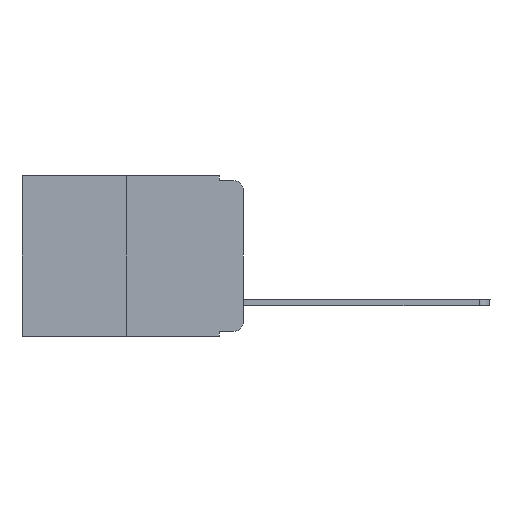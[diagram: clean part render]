
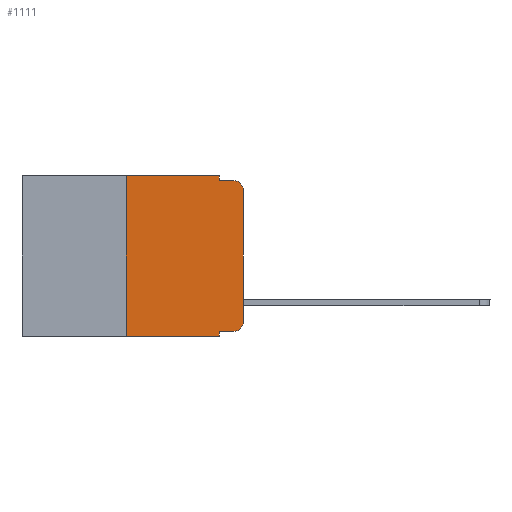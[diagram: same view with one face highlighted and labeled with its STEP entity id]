
A CAD part, left-side view. The second image highlights one B-rep face of the part: STEP entity #1111.
In plain terms, the highlighted planar face has unit normal (-1, 0, 0).
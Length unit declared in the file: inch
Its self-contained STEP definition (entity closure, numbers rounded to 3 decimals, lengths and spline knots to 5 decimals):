
#256 = VERTEX_POINT ( 'NONE', #7959 ) ;
#461 = DIRECTION ( 'NONE',  ( 1., 0., 0. ) ) ;
#579 = VECTOR ( 'NONE', #4716, 39.37008 ) ;
#1111 = ADVANCED_FACE ( 'NONE', ( #8723 ), #7803, .F. ) ;
#1234 = CARTESIAN_POINT ( 'NONE',  ( 0., 0.051, -0.343 ) ) ;
#1401 = LINE ( 'NONE', #1461, #579 ) ;
#1404 = DIRECTION ( 'NONE',  ( 0., 0., 1. ) ) ;
#1461 = CARTESIAN_POINT ( 'NONE',  ( 0., 0.473, -0.343 ) ) ;
#1511 = VECTOR ( 'NONE', #13903, 39.37008 ) ;
#1531 = CARTESIAN_POINT ( 'NONE',  ( 0., 0., 0. ) ) ;
#1601 = LINE ( 'NONE', #1531, #5563 ) ;
#2451 = DIRECTION ( 'NONE',  ( 0., 0., -1. ) ) ;
#2558 = DIRECTION ( 'NONE',  ( 0., -1., 0. ) ) ;
#2693 = CARTESIAN_POINT ( 'NONE',  ( 0., 0.473, 0. ) ) ;
#2708 = CARTESIAN_POINT ( 'NONE',  ( 0., 0.25, -0.343 ) ) ;
#2751 = DIRECTION ( 'NONE',  ( -1., 0., 0. ) ) ;
#3052 = VECTOR ( 'NONE', #9156, 39.37008 ) ;
#3232 = VERTEX_POINT ( 'NONE', #2708 ) ;
#3564 = AXIS2_PLACEMENT_3D ( 'NONE', #12555, #2751, #6198 ) ;
#3729 = CARTESIAN_POINT ( 'NONE',  ( 0., 0.02, -0.333 ) ) ;
#4047 = ORIENTED_EDGE ( 'NONE', *, *, #6464, .F. ) ;
#4077 = LINE ( 'NONE', #13538, #3052 ) ;
#4249 = AXIS2_PLACEMENT_3D ( 'NONE', #7734, #461, #6663 ) ;
#4561 = CARTESIAN_POINT ( 'NONE',  ( 0., 0.02, -0.313 ) ) ;
#4716 = DIRECTION ( 'NONE',  ( 0., -1., 0. ) ) ;
#5084 = CARTESIAN_POINT ( 'NONE',  ( 0., 0.051, -0.01 ) ) ;
#5100 = VECTOR ( 'NONE', #2558, 39.37008 ) ;
#5125 = CARTESIAN_POINT ( 'NONE',  ( 0., 0., -0.03 ) ) ;
#5132 = ORIENTED_EDGE ( 'NONE', *, *, #7488, .F. ) ;
#5205 = CARTESIAN_POINT ( 'NONE',  ( 0., 0.02, -0.01 ) ) ;
#5471 = ORIENTED_EDGE ( 'NONE', *, *, #10365, .T. ) ;
#5563 = VECTOR ( 'NONE', #1404, 39.37008 ) ;
#5579 = EDGE_CURVE ( 'NONE', #12009, #11403, #11857, .T. ) ;
#5603 = AXIS2_PLACEMENT_3D ( 'NONE', #4561, #7944, #2451 ) ;
#6198 = DIRECTION ( 'NONE',  ( 0., 0., -1. ) ) ;
#6370 = EDGE_CURVE ( 'NONE', #256, #7453, #8832, .T. ) ;
#6383 = CARTESIAN_POINT ( 'NONE',  ( 0., 0.051, -0.01 ) ) ;
#6464 = EDGE_CURVE ( 'NONE', #11403, #8611, #9401, .T. ) ;
#6608 = VECTOR ( 'NONE', #9745, 39.37008 ) ;
#6645 = ORIENTED_EDGE ( 'NONE', *, *, #10499, .F. ) ;
#6663 = DIRECTION ( 'NONE',  ( 0., 0., -1. ) ) ;
#6860 = EDGE_CURVE ( 'NONE', #3232, #7453, #1401, .T. ) ;
#6876 = VERTEX_POINT ( 'NONE', #5125 ) ;
#6927 = ORIENTED_EDGE ( 'NONE', *, *, #11075, .T. ) ;
#6972 = VERTEX_POINT ( 'NONE', #9577 ) ;
#7328 = CARTESIAN_POINT ( 'NONE',  ( 0., 0.25, 0. ) ) ;
#7453 = VERTEX_POINT ( 'NONE', #1234 ) ;
#7488 = EDGE_CURVE ( 'NONE', #6972, #12009, #13480, .T. ) ;
#7600 = LINE ( 'NONE', #7328, #1511 ) ;
#7734 = CARTESIAN_POINT ( 'NONE',  ( 0., 0.473, 0. ) ) ;
#7773 = CARTESIAN_POINT ( 'NONE',  ( 0., 0.051, 0. ) ) ;
#7803 = PLANE ( 'NONE',  #4249 ) ;
#7863 = EDGE_CURVE ( 'NONE', #11870, #6876, #1601, .T. ) ;
#7944 = DIRECTION ( 'NONE',  ( -1., 0., 0. ) ) ;
#7954 = VERTEX_POINT ( 'NONE', #3729 ) ;
#7959 = CARTESIAN_POINT ( 'NONE',  ( 0., 0.051, -0.333 ) ) ;
#8611 = VERTEX_POINT ( 'NONE', #5205 ) ;
#8723 = FACE_OUTER_BOUND ( 'NONE', #10861, .T. ) ;
#8832 = LINE ( 'NONE', #7773, #11361 ) ;
#9156 = DIRECTION ( 'NONE',  ( 0., -1., 0. ) ) ;
#9245 = ORIENTED_EDGE ( 'NONE', *, *, #12134, .T. ) ;
#9401 = LINE ( 'NONE', #5084, #10695 ) ;
#9577 = CARTESIAN_POINT ( 'NONE',  ( 0., 0.25, 0. ) ) ;
#9745 = DIRECTION ( 'NONE',  ( 0., 0., -1. ) ) ;
#9897 = CARTESIAN_POINT ( 'NONE',  ( 0., 0.051, 0. ) ) ;
#10037 = DIRECTION ( 'NONE',  ( 0., 0., -1. ) ) ;
#10365 = EDGE_CURVE ( 'NONE', #6876, #8611, #12806, .T. ) ;
#10499 = EDGE_CURVE ( 'NONE', #3232, #6972, #7600, .T. ) ;
#10695 = VECTOR ( 'NONE', #12431, 39.37008 ) ;
#10861 = EDGE_LOOP ( 'NONE', ( #13128, #5471, #4047, #13008, #5132, #6645, #11641, #13350, #9245, #6927 ) ) ;
#11075 = EDGE_CURVE ( 'NONE', #7954, #11870, #11699, .T. ) ;
#11361 = VECTOR ( 'NONE', #10037, 39.37008 ) ;
#11403 = VERTEX_POINT ( 'NONE', #6383 ) ;
#11611 = CARTESIAN_POINT ( 'NONE',  ( 0., 0., -0.313 ) ) ;
#11641 = ORIENTED_EDGE ( 'NONE', *, *, #6860, .T. ) ;
#11699 = CIRCLE ( 'NONE', #5603, 0.02 ) ;
#11790 = CARTESIAN_POINT ( 'NONE',  ( 0., 0.051, 0. ) ) ;
#11857 = LINE ( 'NONE', #11790, #6608 ) ;
#11870 = VERTEX_POINT ( 'NONE', #11611 ) ;
#12009 = VERTEX_POINT ( 'NONE', #9897 ) ;
#12134 = EDGE_CURVE ( 'NONE', #256, #7954, #4077, .T. ) ;
#12431 = DIRECTION ( 'NONE',  ( 0., -1., 0. ) ) ;
#12555 = CARTESIAN_POINT ( 'NONE',  ( 0., 0.02, -0.03 ) ) ;
#12806 = CIRCLE ( 'NONE', #3564, 0.02 ) ;
#13008 = ORIENTED_EDGE ( 'NONE', *, *, #5579, .F. ) ;
#13128 = ORIENTED_EDGE ( 'NONE', *, *, #7863, .T. ) ;
#13350 = ORIENTED_EDGE ( 'NONE', *, *, #6370, .F. ) ;
#13480 = LINE ( 'NONE', #2693, #5100 ) ;
#13538 = CARTESIAN_POINT ( 'NONE',  ( 0., 0.051, -0.333 ) ) ;
#13903 = DIRECTION ( 'NONE',  ( 0., 0., 1. ) ) ;
